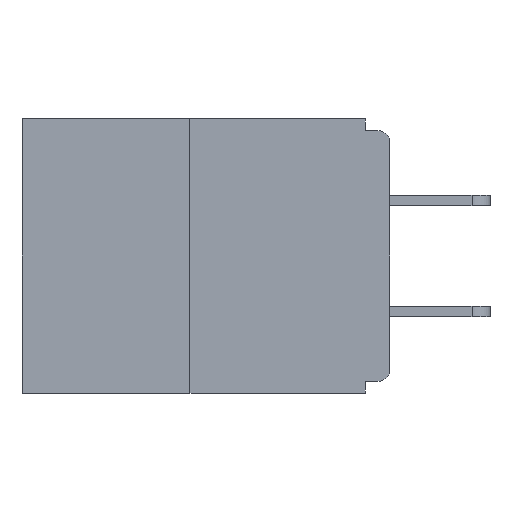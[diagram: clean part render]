
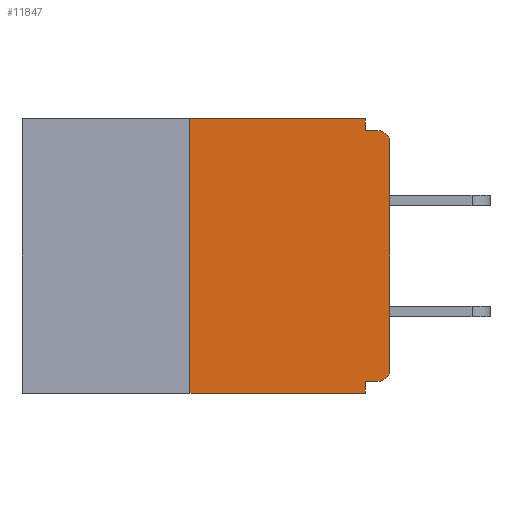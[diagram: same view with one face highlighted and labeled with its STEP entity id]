
A CAD part, left-side view. The second image highlights one B-rep face of the part: STEP entity #11847.
In plain terms, the highlighted planar face has unit normal (-1, 0, 0).
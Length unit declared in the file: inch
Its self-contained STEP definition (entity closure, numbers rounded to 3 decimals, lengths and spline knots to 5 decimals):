
#62 = VECTOR ( 'NONE', #5865, 39.37008 ) ;
#149 = VECTOR ( 'NONE', #13601, 39.37008 ) ;
#277 = DIRECTION ( 'NONE',  ( 0., -1., 0. ) ) ;
#1077 = VERTEX_POINT ( 'NONE', #9508 ) ;
#1179 = CARTESIAN_POINT ( 'NONE',  ( 0., 0., 0. ) ) ;
#1422 = DIRECTION ( 'NONE',  ( 0., 1., 0. ) ) ;
#1745 = ORIENTED_EDGE ( 'NONE', *, *, #2031, .T. ) ;
#1932 = LINE ( 'NONE', #10246, #9124 ) ;
#1999 = VERTEX_POINT ( 'NONE', #16710 ) ;
#2031 = EDGE_CURVE ( 'NONE', #4560, #4132, #16950, .T. ) ;
#2080 = ORIENTED_EDGE ( 'NONE', *, *, #8165, .F. ) ;
#2170 = DIRECTION ( 'NONE',  ( 0., 0., -1. ) ) ;
#2401 = LINE ( 'NONE', #1179, #13839 ) ;
#2936 = LINE ( 'NONE', #9518, #6034 ) ;
#3338 = CARTESIAN_POINT ( 'NONE',  ( 0., 0.46, 0. ) ) ;
#3705 = CARTESIAN_POINT ( 'NONE',  ( 0., 0.031, -0.015 ) ) ;
#4132 = VERTEX_POINT ( 'NONE', #10769 ) ;
#4352 = CARTESIAN_POINT ( 'NONE',  ( 0., 0.031, 0. ) ) ;
#4560 = VERTEX_POINT ( 'NONE', #16309 ) ;
#4569 = DIRECTION ( 'NONE',  ( 1., 0., 0. ) ) ;
#4663 = CARTESIAN_POINT ( 'NONE',  ( 0., 0., -0.03 ) ) ;
#4683 = DIRECTION ( 'NONE',  ( 0., 0., -1. ) ) ;
#4861 = VECTOR ( 'NONE', #1422, 39.37008 ) ;
#4987 = ORIENTED_EDGE ( 'NONE', *, *, #6732, .T. ) ;
#5030 = CARTESIAN_POINT ( 'NONE',  ( 0., 0., -0.328 ) ) ;
#5089 = EDGE_CURVE ( 'NONE', #6912, #14856, #11414, .T. ) ;
#5235 = LINE ( 'NONE', #9898, #62 ) ;
#5571 = EDGE_CURVE ( 'NONE', #1999, #16601, #8177, .T. ) ;
#5865 = DIRECTION ( 'NONE',  ( 0., -1., 0. ) ) ;
#5879 = PLANE ( 'NONE',  #13462 ) ;
#5990 = EDGE_LOOP ( 'NONE', ( #2080, #7898, #1745, #10252, #7480, #4987, #7943, #15768, #13491, #9178 ) ) ;
#6019 = CARTESIAN_POINT ( 'NONE',  ( 0., 0.031, -0.343 ) ) ;
#6034 = VECTOR ( 'NONE', #277, 39.37008 ) ;
#6732 = EDGE_CURVE ( 'NONE', #10551, #1077, #11187, .T. ) ;
#6804 = EDGE_CURVE ( 'NONE', #10551, #7346, #11769, .T. ) ;
#6912 = VERTEX_POINT ( 'NONE', #4663 ) ;
#7077 = CARTESIAN_POINT ( 'NONE',  ( 0., 0.25, 0. ) ) ;
#7097 = CARTESIAN_POINT ( 'NONE',  ( 0., 0.015, -0.328 ) ) ;
#7346 = VERTEX_POINT ( 'NONE', #11780 ) ;
#7480 = ORIENTED_EDGE ( 'NONE', *, *, #6804, .F. ) ;
#7713 = AXIS2_PLACEMENT_3D ( 'NONE', #15183, #8757, #2170 ) ;
#7898 = ORIENTED_EDGE ( 'NONE', *, *, #11239, .F. ) ;
#7943 = ORIENTED_EDGE ( 'NONE', *, *, #14993, .T. ) ;
#8165 = EDGE_CURVE ( 'NONE', #9067, #1999, #2936, .T. ) ;
#8177 = LINE ( 'NONE', #4352, #149 ) ;
#8757 = DIRECTION ( 'NONE',  ( -1., 0., 0. ) ) ;
#8828 = CARTESIAN_POINT ( 'NONE',  ( 0., 0.015, -0.313 ) ) ;
#8831 = VECTOR ( 'NONE', #15255, 39.37008 ) ;
#8876 = VECTOR ( 'NONE', #16779, 39.37008 ) ;
#8985 = CARTESIAN_POINT ( 'NONE',  ( 0., 0.015, -0.015 ) ) ;
#9067 = VERTEX_POINT ( 'NONE', #7077 ) ;
#9124 = VECTOR ( 'NONE', #10139, 39.37008 ) ;
#9178 = ORIENTED_EDGE ( 'NONE', *, *, #5571, .F. ) ;
#9198 = EDGE_CURVE ( 'NONE', #7346, #4132, #16589, .T. ) ;
#9508 = CARTESIAN_POINT ( 'NONE',  ( 0., 0., -0.313 ) ) ;
#9518 = CARTESIAN_POINT ( 'NONE',  ( 0., 0.46, 0. ) ) ;
#9898 = CARTESIAN_POINT ( 'NONE',  ( 0., 0., -0.015 ) ) ;
#10139 = DIRECTION ( 'NONE',  ( 0., 0., 1. ) ) ;
#10246 = CARTESIAN_POINT ( 'NONE',  ( 0., 0.25, 0. ) ) ;
#10252 = ORIENTED_EDGE ( 'NONE', *, *, #9198, .F. ) ;
#10551 = VERTEX_POINT ( 'NONE', #7097 ) ;
#10769 = CARTESIAN_POINT ( 'NONE',  ( 0., 0.031, -0.343 ) ) ;
#11187 = CIRCLE ( 'NONE', #14558, 0.015 ) ;
#11239 = EDGE_CURVE ( 'NONE', #4560, #9067, #1932, .T. ) ;
#11249 = DIRECTION ( 'NONE',  ( -1., 0., 0. ) ) ;
#11406 = CARTESIAN_POINT ( 'NONE',  ( 0., 0.46, -0.343 ) ) ;
#11414 = CIRCLE ( 'NONE', #7713, 0.015 ) ;
#11769 = LINE ( 'NONE', #5030, #4861 ) ;
#11780 = CARTESIAN_POINT ( 'NONE',  ( 0., 0.031, -0.328 ) ) ;
#11847 = ADVANCED_FACE ( 'NONE', ( #12745 ), #5879, .F. ) ;
#12169 = EDGE_CURVE ( 'NONE', #16601, #14856, #5235, .T. ) ;
#12745 = FACE_OUTER_BOUND ( 'NONE', #5990, .T. ) ;
#13462 = AXIS2_PLACEMENT_3D ( 'NONE', #3338, #4569, #4683 ) ;
#13491 = ORIENTED_EDGE ( 'NONE', *, *, #12169, .F. ) ;
#13601 = DIRECTION ( 'NONE',  ( 0., 0., -1. ) ) ;
#13839 = VECTOR ( 'NONE', #16698, 39.37008 ) ;
#14558 = AXIS2_PLACEMENT_3D ( 'NONE', #8828, #11249, #15362 ) ;
#14856 = VERTEX_POINT ( 'NONE', #8985 ) ;
#14993 = EDGE_CURVE ( 'NONE', #1077, #6912, #2401, .T. ) ;
#15183 = CARTESIAN_POINT ( 'NONE',  ( 0., 0.015, -0.03 ) ) ;
#15255 = DIRECTION ( 'NONE',  ( 0., -1., 0. ) ) ;
#15362 = DIRECTION ( 'NONE',  ( 0., 0., -1. ) ) ;
#15768 = ORIENTED_EDGE ( 'NONE', *, *, #5089, .T. ) ;
#16309 = CARTESIAN_POINT ( 'NONE',  ( 0., 0.25, -0.343 ) ) ;
#16589 = LINE ( 'NONE', #6019, #8876 ) ;
#16601 = VERTEX_POINT ( 'NONE', #3705 ) ;
#16698 = DIRECTION ( 'NONE',  ( 0., 0., 1. ) ) ;
#16710 = CARTESIAN_POINT ( 'NONE',  ( 0., 0.031, 0. ) ) ;
#16779 = DIRECTION ( 'NONE',  ( 0., 0., -1. ) ) ;
#16950 = LINE ( 'NONE', #11406, #8831 ) ;
